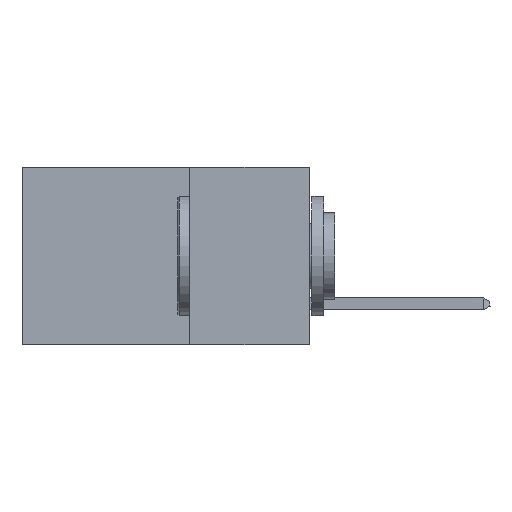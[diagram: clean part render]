
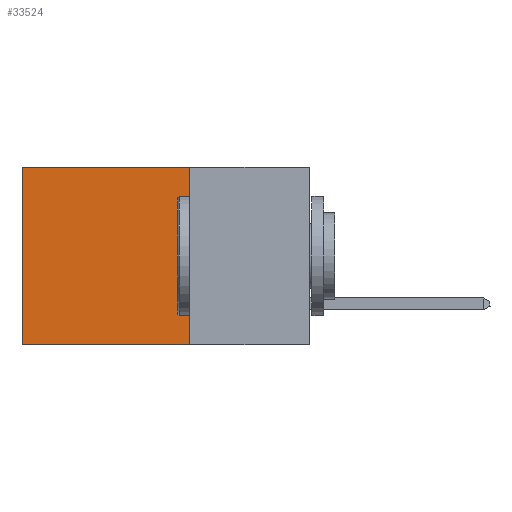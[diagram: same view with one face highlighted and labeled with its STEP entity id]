
A CAD part, left-side view. The second image highlights one B-rep face of the part: STEP entity #33524.
In plain terms, the highlighted planar face has unit normal (-1, 0, 0).
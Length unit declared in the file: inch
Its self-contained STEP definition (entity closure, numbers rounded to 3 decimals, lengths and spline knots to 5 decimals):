
#1141 = CARTESIAN_POINT ( 'NONE',  ( 0.2875, 0.6, 0. ) ) ;
#2933 = VERTEX_POINT ( 'NONE', #32239 ) ;
#5576 = CARTESIAN_POINT ( 'NONE',  ( 0.2875, 0.25, 0. ) ) ;
#6252 = CARTESIAN_POINT ( 'NONE',  ( 0.2875, 0.25, -0.37 ) ) ;
#7236 = DIRECTION ( 'NONE',  ( 0., 0., -1. ) ) ;
#7319 = EDGE_CURVE ( 'NONE', #2933, #8277, #28378, .T. ) ;
#7372 = ORIENTED_EDGE ( 'NONE', *, *, #7319, .T. ) ;
#7884 = VERTEX_POINT ( 'NONE', #21533 ) ;
#8277 = VERTEX_POINT ( 'NONE', #47472 ) ;
#9256 = FACE_OUTER_BOUND ( 'NONE', #19044, .T. ) ;
#13865 = EDGE_CURVE ( 'NONE', #28308, #7884, #26271, .T. ) ;
#13908 = DIRECTION ( 'NONE',  ( 0., 1., 0. ) ) ;
#14516 = LINE ( 'NONE', #6252, #31975 ) ;
#16616 = AXIS2_PLACEMENT_3D ( 'NONE', #45810, #27211, #20370 ) ;
#19044 = EDGE_LOOP ( 'NONE', ( #7372, #43737, #19262, #45137 ) ) ;
#19262 = ORIENTED_EDGE ( 'NONE', *, *, #13865, .F. ) ;
#20370 = DIRECTION ( 'NONE',  ( 0., 0., -1. ) ) ;
#21008 = CARTESIAN_POINT ( 'NONE',  ( 0.2875, 0.25, 0. ) ) ;
#21533 = CARTESIAN_POINT ( 'NONE',  ( 0.2875, 0.25, -0.37 ) ) ;
#23764 = EDGE_CURVE ( 'NONE', #28308, #2933, #47676, .T. ) ;
#23890 = VECTOR ( 'NONE', #7236, 39.37008 ) ;
#24578 = DIRECTION ( 'NONE',  ( 0., 1., 0. ) ) ;
#24879 = CARTESIAN_POINT ( 'NONE',  ( 0.2875, 0.25, 0. ) ) ;
#25052 = DIRECTION ( 'NONE',  ( 0., 0., -1. ) ) ;
#26271 = LINE ( 'NONE', #24879, #23890 ) ;
#27211 = DIRECTION ( 'NONE',  ( 1., 0., 0. ) ) ;
#27734 = VECTOR ( 'NONE', #24578, 39.37008 ) ;
#28308 = VERTEX_POINT ( 'NONE', #5576 ) ;
#28378 = LINE ( 'NONE', #1141, #31840 ) ;
#30787 = PLANE ( 'NONE',  #16616 ) ;
#31840 = VECTOR ( 'NONE', #25052, 39.37008 ) ;
#31975 = VECTOR ( 'NONE', #13908, 39.37008 ) ;
#32239 = CARTESIAN_POINT ( 'NONE',  ( 0.2875, 0.6, 0. ) ) ;
#33524 = ADVANCED_FACE ( 'NONE', ( #9256 ), #30787, .F. ) ;
#35162 = EDGE_CURVE ( 'NONE', #7884, #8277, #14516, .T. ) ;
#43737 = ORIENTED_EDGE ( 'NONE', *, *, #35162, .F. ) ;
#45137 = ORIENTED_EDGE ( 'NONE', *, *, #23764, .T. ) ;
#45810 = CARTESIAN_POINT ( 'NONE',  ( 0.2875, 0.25, 0. ) ) ;
#47472 = CARTESIAN_POINT ( 'NONE',  ( 0.2875, 0.6, -0.37 ) ) ;
#47676 = LINE ( 'NONE', #21008, #27734 ) ;
